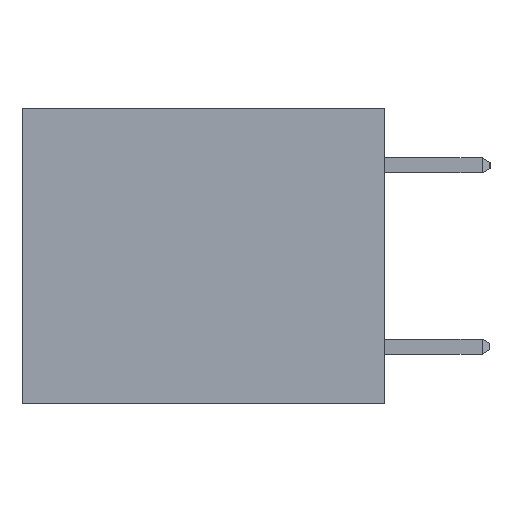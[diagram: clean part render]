
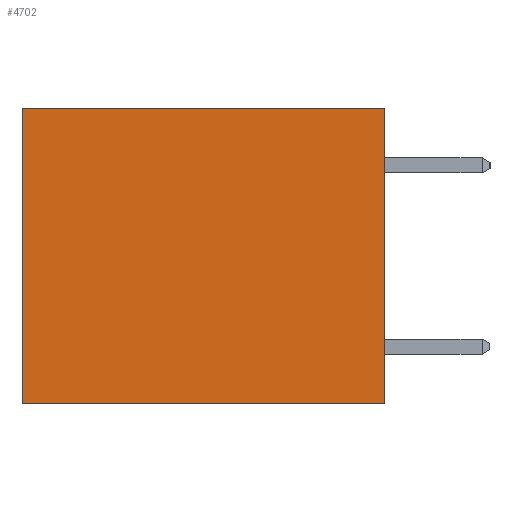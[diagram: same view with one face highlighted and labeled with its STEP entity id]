
A CAD part, left-side view. The second image highlights one B-rep face of the part: STEP entity #4702.
In plain terms, the highlighted planar face has unit normal (-1, 0, 0).
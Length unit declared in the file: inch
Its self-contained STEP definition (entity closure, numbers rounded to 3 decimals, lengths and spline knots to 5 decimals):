
#1446 = DIRECTION ( 'NONE',  ( 0., 1., 0. ) ) ;
#1627 = VECTOR ( 'NONE', #1446, 39.37008 ) ;
#1833 = LINE ( 'NONE', #7350, #9177 ) ;
#2017 = DIRECTION ( 'NONE',  ( 0., 0., -1. ) ) ;
#2212 = CARTESIAN_POINT ( 'NONE',  ( 0.3165, 0.6, -0.49 ) ) ;
#2669 = LINE ( 'NONE', #2212, #8350 ) ;
#2746 = VERTEX_POINT ( 'NONE', #12063 ) ;
#3129 = ORIENTED_EDGE ( 'NONE', *, *, #5479, .T. ) ;
#3830 = DIRECTION ( 'NONE',  ( 0., 0., -1. ) ) ;
#4360 = VECTOR ( 'NONE', #2017, 39.37008 ) ;
#4684 = EDGE_CURVE ( 'NONE', #7489, #2746, #9425, .T. ) ;
#4702 = ADVANCED_FACE ( 'NONE', ( #5408 ), #5755, .F. ) ;
#5064 = CARTESIAN_POINT ( 'NONE',  ( 0.3165, 0.6, -0.49 ) ) ;
#5408 = FACE_OUTER_BOUND ( 'NONE', #7989, .T. ) ;
#5479 = EDGE_CURVE ( 'NONE', #6772, #11817, #2669, .T. ) ;
#5755 = PLANE ( 'NONE',  #8879 ) ;
#6140 = ORIENTED_EDGE ( 'NONE', *, *, #8671, .T. ) ;
#6772 = VERTEX_POINT ( 'NONE', #10289 ) ;
#6784 = EDGE_CURVE ( 'NONE', #2746, #11817, #1833, .T. ) ;
#6799 = CARTESIAN_POINT ( 'NONE',  ( 0.3165, 0., -0.49 ) ) ;
#7192 = CARTESIAN_POINT ( 'NONE',  ( 0.3165, 0., 0. ) ) ;
#7350 = CARTESIAN_POINT ( 'NONE',  ( 0.3165, 0., -0.49 ) ) ;
#7489 = VERTEX_POINT ( 'NONE', #10024 ) ;
#7705 = DIRECTION ( 'NONE',  ( 1., 0., 0. ) ) ;
#7989 = EDGE_LOOP ( 'NONE', ( #3129, #11375, #11624, #6140 ) ) ;
#8350 = VECTOR ( 'NONE', #3830, 39.37008 ) ;
#8671 = EDGE_CURVE ( 'NONE', #7489, #6772, #12236, .T. ) ;
#8879 = AXIS2_PLACEMENT_3D ( 'NONE', #9497, #7705, #10591 ) ;
#9177 = VECTOR ( 'NONE', #9307, 39.37008 ) ;
#9307 = DIRECTION ( 'NONE',  ( 0., 1., 0. ) ) ;
#9425 = LINE ( 'NONE', #6799, #4360 ) ;
#9497 = CARTESIAN_POINT ( 'NONE',  ( 0.3165, 0., -0.49 ) ) ;
#10024 = CARTESIAN_POINT ( 'NONE',  ( 0.3165, 0., 0. ) ) ;
#10289 = CARTESIAN_POINT ( 'NONE',  ( 0.3165, 0.6, 0. ) ) ;
#10591 = DIRECTION ( 'NONE',  ( 0., 0., -1. ) ) ;
#11375 = ORIENTED_EDGE ( 'NONE', *, *, #6784, .F. ) ;
#11624 = ORIENTED_EDGE ( 'NONE', *, *, #4684, .F. ) ;
#11817 = VERTEX_POINT ( 'NONE', #5064 ) ;
#12063 = CARTESIAN_POINT ( 'NONE',  ( 0.3165, 0., -0.49 ) ) ;
#12236 = LINE ( 'NONE', #7192, #1627 ) ;
